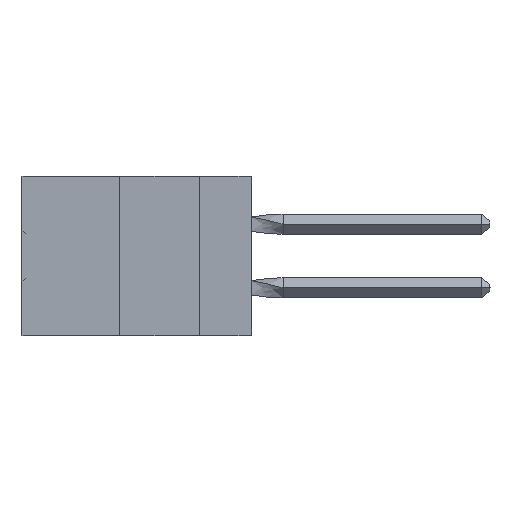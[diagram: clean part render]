
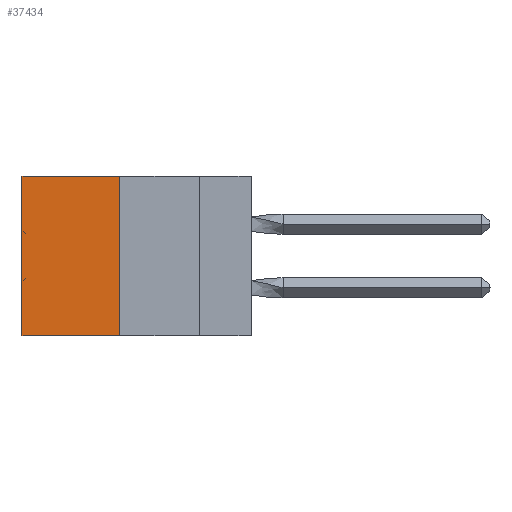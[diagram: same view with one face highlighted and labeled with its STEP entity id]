
A CAD part, left-side view. The second image highlights one B-rep face of the part: STEP entity #37434.
In plain terms, the highlighted planar face has unit normal (-1, 0, 0).
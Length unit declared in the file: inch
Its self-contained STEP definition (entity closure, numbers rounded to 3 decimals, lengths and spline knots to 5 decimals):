
#5188 = LINE ( 'NONE', #26269, #33232 ) ;
#5352 = VECTOR ( 'NONE', #33009, 39.37008 ) ;
#8532 = CARTESIAN_POINT ( 'NONE',  ( 0.305, 0.413, -0.5 ) ) ;
#8927 = EDGE_CURVE ( 'NONE', #26841, #32068, #42516, .T. ) ;
#10303 = EDGE_CURVE ( 'NONE', #40209, #36068, #5188, .T. ) ;
#12634 = VECTOR ( 'NONE', #35637, 39.37008 ) ;
#13638 = LINE ( 'NONE', #27031, #35351 ) ;
#14930 = CARTESIAN_POINT ( 'NONE',  ( 0.305, 0.413, 0. ) ) ;
#15067 = EDGE_LOOP ( 'NONE', ( #39610, #47602, #47965, #47192 ) ) ;
#24464 = DIRECTION ( 'NONE',  ( 0., 0., -1. ) ) ;
#24657 = CARTESIAN_POINT ( 'NONE',  ( 0.305, 0.413, -0.5 ) ) ;
#26269 = CARTESIAN_POINT ( 'NONE',  ( 0.305, 0.413, -0.5 ) ) ;
#26841 = VERTEX_POINT ( 'NONE', #53026 ) ;
#27031 = CARTESIAN_POINT ( 'NONE',  ( 0.305, 0.413, 0. ) ) ;
#28128 = CARTESIAN_POINT ( 'NONE',  ( 0.305, 0.72, -0.5 ) ) ;
#32068 = VERTEX_POINT ( 'NONE', #52809 ) ;
#32220 = LINE ( 'NONE', #49114, #12634 ) ;
#33009 = DIRECTION ( 'NONE',  ( 0., 0., -1. ) ) ;
#33232 = VECTOR ( 'NONE', #34534, 39.37008 ) ;
#33731 = PLANE ( 'NONE',  #38739 ) ;
#34534 = DIRECTION ( 'NONE',  ( 0., 0., -1. ) ) ;
#35351 = VECTOR ( 'NONE', #40010, 39.37008 ) ;
#35637 = DIRECTION ( 'NONE',  ( 0., 1., 0. ) ) ;
#36068 = VERTEX_POINT ( 'NONE', #8532 ) ;
#37434 = ADVANCED_FACE ( 'NONE', ( #47922 ), #33731, .F. ) ;
#38739 = AXIS2_PLACEMENT_3D ( 'NONE', #24657, #42552, #24464 ) ;
#39610 = ORIENTED_EDGE ( 'NONE', *, *, #8927, .T. ) ;
#40010 = DIRECTION ( 'NONE',  ( 0., 1., 0. ) ) ;
#40209 = VERTEX_POINT ( 'NONE', #14930 ) ;
#42516 = LINE ( 'NONE', #28128, #5352 ) ;
#42552 = DIRECTION ( 'NONE',  ( 1., 0., 0. ) ) ;
#46698 = EDGE_CURVE ( 'NONE', #40209, #26841, #13638, .T. ) ;
#47192 = ORIENTED_EDGE ( 'NONE', *, *, #46698, .T. ) ;
#47602 = ORIENTED_EDGE ( 'NONE', *, *, #52550, .F. ) ;
#47922 = FACE_OUTER_BOUND ( 'NONE', #15067, .T. ) ;
#47965 = ORIENTED_EDGE ( 'NONE', *, *, #10303, .F. ) ;
#49114 = CARTESIAN_POINT ( 'NONE',  ( 0.305, 0.413, -0.5 ) ) ;
#52550 = EDGE_CURVE ( 'NONE', #36068, #32068, #32220, .T. ) ;
#52809 = CARTESIAN_POINT ( 'NONE',  ( 0.305, 0.72, -0.5 ) ) ;
#53026 = CARTESIAN_POINT ( 'NONE',  ( 0.305, 0.72, 0. ) ) ;
